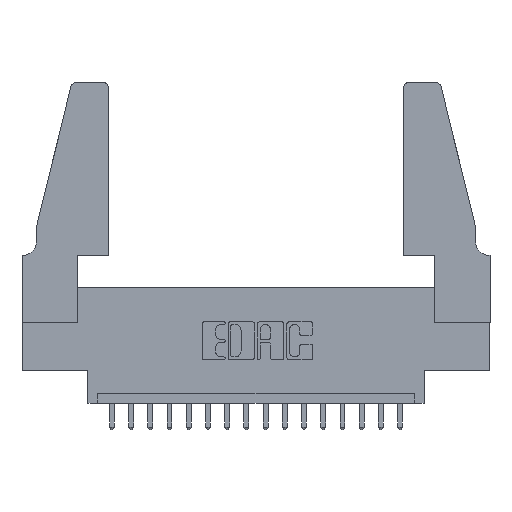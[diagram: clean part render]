
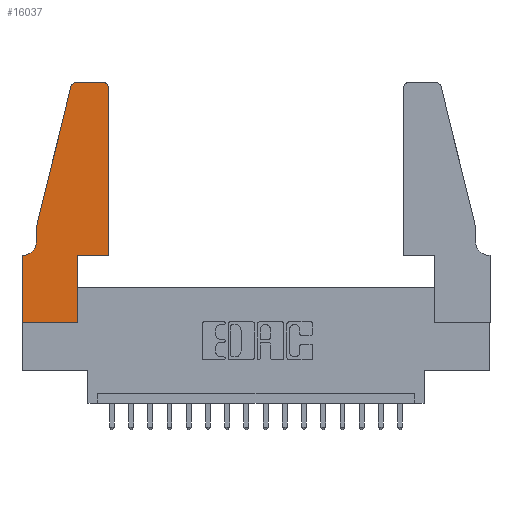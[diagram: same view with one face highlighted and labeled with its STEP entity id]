
A CAD part, top view. The second image highlights one B-rep face of the part: STEP entity #16037.
In plain terms, the highlighted planar face has unit normal (0, 0, 1).
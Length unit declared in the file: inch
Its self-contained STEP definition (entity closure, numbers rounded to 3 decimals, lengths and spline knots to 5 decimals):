
#334 = EDGE_CURVE ( 'NONE', #14171, #17834, #2341, .T. ) ;
#371 = LINE ( 'NONE', #10965, #15920 ) ;
#443 = DIRECTION ( 'NONE',  ( 0., 0., 1. ) ) ;
#631 = CARTESIAN_POINT ( 'NONE',  ( 0., 0., 0.37 ) ) ;
#970 = EDGE_CURVE ( 'NONE', #2568, #14171, #9013, .T. ) ;
#1109 = EDGE_CURVE ( 'NONE', #14676, #8653, #14400, .T. ) ;
#1214 = VECTOR ( 'NONE', #17433, 39.37008 ) ;
#1312 = VECTOR ( 'NONE', #7545, 39.37008 ) ;
#1336 = CARTESIAN_POINT ( 'NONE',  ( 0.0755, 0.42, 0.37 ) ) ;
#1371 = EDGE_CURVE ( 'NONE', #17834, #6579, #16340, .T. ) ;
#1419 = DIRECTION ( 'NONE',  ( 0., 1., 0. ) ) ;
#1671 = DIRECTION ( 'NONE',  ( 0., 0., -1. ) ) ;
#1838 = ORIENTED_EDGE ( 'NONE', *, *, #9857, .T. ) ;
#1872 = VECTOR ( 'NONE', #6189, 39.37008 ) ;
#1971 = VECTOR ( 'NONE', #13880, 39.37008 ) ;
#2239 = ORIENTED_EDGE ( 'NONE', *, *, #5263, .T. ) ;
#2341 = CIRCLE ( 'NONE', #7949, 0.03 ) ;
#2568 = VERTEX_POINT ( 'NONE', #13016 ) ;
#2599 = CARTESIAN_POINT ( 'NONE',  ( 0.4205, 1.25, 0.37 ) ) ;
#2701 = DIRECTION ( 'NONE',  ( -1., 0., 0. ) ) ;
#2785 = ORIENTED_EDGE ( 'NONE', *, *, #7312, .T. ) ;
#2847 = ORIENTED_EDGE ( 'NONE', *, *, #6671, .T. ) ;
#3086 = LINE ( 'NONE', #13946, #1971 ) ;
#3127 = VERTEX_POINT ( 'NONE', #8955 ) ;
#3413 = CARTESIAN_POINT ( 'NONE',  ( 0.4505, 0.35, 0.37 ) ) ;
#3424 = LINE ( 'NONE', #14992, #8168 ) ;
#4286 = CARTESIAN_POINT ( 'NONE',  ( 0., 0.35, 0.37 ) ) ;
#4294 = ORIENTED_EDGE ( 'NONE', *, *, #970, .T. ) ;
#5222 = ORIENTED_EDGE ( 'NONE', *, *, #9639, .T. ) ;
#5263 = EDGE_CURVE ( 'NONE', #8653, #3127, #8432, .T. ) ;
#5551 = CARTESIAN_POINT ( 'NONE',  ( 0.284, 1.25, 0.37 ) ) ;
#5557 = EDGE_CURVE ( 'NONE', #3127, #13647, #6450, .T. ) ;
#5804 = DIRECTION ( 'NONE',  ( -1., 0., 0. ) ) ;
#6171 = EDGE_CURVE ( 'NONE', #14472, #9930, #13128, .T. ) ;
#6189 = DIRECTION ( 'NONE',  ( 0., 1., 0. ) ) ;
#6231 = CARTESIAN_POINT ( 'NONE',  ( 0.0755, 0.5, 0.37 ) ) ;
#6242 = VECTOR ( 'NONE', #1419, 39.37008 ) ;
#6450 = LINE ( 'NONE', #12397, #6242 ) ;
#6579 = VERTEX_POINT ( 'NONE', #5551 ) ;
#6671 = EDGE_CURVE ( 'NONE', #6579, #7304, #11399, .T. ) ;
#6766 = ORIENTED_EDGE ( 'NONE', *, *, #334, .T. ) ;
#7304 = VERTEX_POINT ( 'NONE', #15136 ) ;
#7312 = EDGE_CURVE ( 'NONE', #9930, #14676, #371, .T. ) ;
#7545 = DIRECTION ( 'NONE',  ( 1., 0., 0. ) ) ;
#7598 = ORIENTED_EDGE ( 'NONE', *, *, #1109, .T. ) ;
#7949 = AXIS2_PLACEMENT_3D ( 'NONE', #12731, #443, #8524 ) ;
#8168 = VECTOR ( 'NONE', #10825, 39.37008 ) ;
#8432 = LINE ( 'NONE', #15826, #1312 ) ;
#8524 = DIRECTION ( 'NONE',  ( 1., 0., 0. ) ) ;
#8653 = VERTEX_POINT ( 'NONE', #631 ) ;
#8951 = EDGE_LOOP ( 'NONE', ( #14739, #2847, #14031, #5222, #15538, #2785, #7598, #2239, #13045, #1838, #4294, #6766 ) ) ;
#8955 = CARTESIAN_POINT ( 'NONE',  ( 0.2865, 0., 0.37 ) ) ;
#9013 = LINE ( 'NONE', #3413, #1872 ) ;
#9639 = EDGE_CURVE ( 'NONE', #13228, #14472, #3086, .T. ) ;
#9659 = DIRECTION ( 'NONE',  ( -1., 0., 0. ) ) ;
#9726 = CARTESIAN_POINT ( 'NONE',  ( 0.2605, 1.25, 0.37 ) ) ;
#9786 = DIRECTION ( 'NONE',  ( 1., 0., 0. ) ) ;
#9857 = EDGE_CURVE ( 'NONE', #13647, #2568, #14091, .T. ) ;
#9930 = VERTEX_POINT ( 'NONE', #11581 ) ;
#10034 = PLANE ( 'NONE',  #16712 ) ;
#10825 = DIRECTION ( 'NONE',  ( -0.239, -0.971, 0. ) ) ;
#10965 = CARTESIAN_POINT ( 'NONE',  ( 0.0755, 0.35, 0.37 ) ) ;
#11118 = CARTESIAN_POINT ( 'NONE',  ( 0., 0.35, 0.37 ) ) ;
#11399 = CIRCLE ( 'NONE', #12522, 0.03 ) ;
#11581 = CARTESIAN_POINT ( 'NONE',  ( 0.0055, 0.35, 0.37 ) ) ;
#11998 = CARTESIAN_POINT ( 'NONE',  ( 0., 0., 0.37 ) ) ;
#12397 = CARTESIAN_POINT ( 'NONE',  ( 0.2865, 0.35, 0.37 ) ) ;
#12522 = AXIS2_PLACEMENT_3D ( 'NONE', #16679, #14018, #15433 ) ;
#12703 = CARTESIAN_POINT ( 'NONE',  ( 0.0055, 0.42, 0.37 ) ) ;
#12731 = CARTESIAN_POINT ( 'NONE',  ( 0.4205, 1.22, 0.37 ) ) ;
#12778 = VECTOR ( 'NONE', #9786, 39.37008 ) ;
#13016 = CARTESIAN_POINT ( 'NONE',  ( 0.4505, 0.35, 0.37 ) ) ;
#13045 = ORIENTED_EDGE ( 'NONE', *, *, #5557, .T. ) ;
#13128 = CIRCLE ( 'NONE', #14825, 0.07 ) ;
#13228 = VERTEX_POINT ( 'NONE', #6231 ) ;
#13647 = VERTEX_POINT ( 'NONE', #16920 ) ;
#13880 = DIRECTION ( 'NONE',  ( 0., -1., 0. ) ) ;
#13883 = CARTESIAN_POINT ( 'NONE',  ( 0.4505, 0.35, 0.37 ) ) ;
#13946 = CARTESIAN_POINT ( 'NONE',  ( 0.0755, 0.5, 0.37 ) ) ;
#14018 = DIRECTION ( 'NONE',  ( 0., 0., 1. ) ) ;
#14031 = ORIENTED_EDGE ( 'NONE', *, *, #14928, .T. ) ;
#14091 = LINE ( 'NONE', #13883, #12778 ) ;
#14171 = VERTEX_POINT ( 'NONE', #15029 ) ;
#14400 = LINE ( 'NONE', #11998, #1214 ) ;
#14472 = VERTEX_POINT ( 'NONE', #1336 ) ;
#14613 = FACE_OUTER_BOUND ( 'NONE', #8951, .T. ) ;
#14676 = VERTEX_POINT ( 'NONE', #4286 ) ;
#14739 = ORIENTED_EDGE ( 'NONE', *, *, #1371, .T. ) ;
#14825 = AXIS2_PLACEMENT_3D ( 'NONE', #12703, #1671, #5804 ) ;
#14928 = EDGE_CURVE ( 'NONE', #7304, #13228, #3424, .T. ) ;
#14992 = CARTESIAN_POINT ( 'NONE',  ( 0.0755, 0.5, 0.37 ) ) ;
#15029 = CARTESIAN_POINT ( 'NONE',  ( 0.4505, 1.22, 0.37 ) ) ;
#15136 = CARTESIAN_POINT ( 'NONE',  ( 0.25487, 1.22718, 0.37 ) ) ;
#15288 = DIRECTION ( 'NONE',  ( 1., 0., 0. ) ) ;
#15354 = DIRECTION ( 'NONE',  ( 0., 0., 1. ) ) ;
#15433 = DIRECTION ( 'NONE',  ( 1., 0., 0. ) ) ;
#15538 = ORIENTED_EDGE ( 'NONE', *, *, #6171, .T. ) ;
#15826 = CARTESIAN_POINT ( 'NONE',  ( 0., 0., 0.37 ) ) ;
#15920 = VECTOR ( 'NONE', #2701, 39.37008 ) ;
#16037 = ADVANCED_FACE ( 'NONE', ( #14613 ), #10034, .T. ) ;
#16340 = LINE ( 'NONE', #9726, #16972 ) ;
#16679 = CARTESIAN_POINT ( 'NONE',  ( 0.284, 1.22, 0.37 ) ) ;
#16712 = AXIS2_PLACEMENT_3D ( 'NONE', #11118, #15354, #15288 ) ;
#16920 = CARTESIAN_POINT ( 'NONE',  ( 0.2865, 0.35, 0.37 ) ) ;
#16972 = VECTOR ( 'NONE', #9659, 39.37008 ) ;
#17433 = DIRECTION ( 'NONE',  ( 0., -1., 0. ) ) ;
#17834 = VERTEX_POINT ( 'NONE', #2599 ) ;
